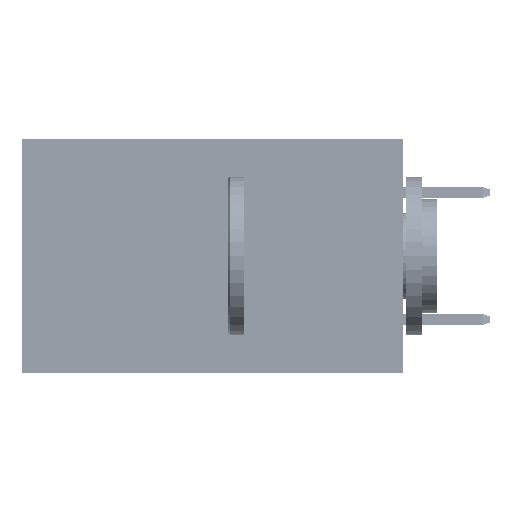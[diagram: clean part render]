
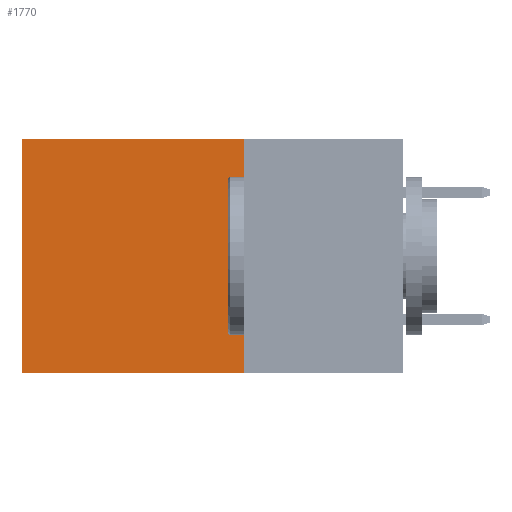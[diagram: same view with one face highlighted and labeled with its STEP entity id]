
A CAD part, left-side view. The second image highlights one B-rep face of the part: STEP entity #1770.
In plain terms, the highlighted planar face has unit normal (-1, 0, 0).
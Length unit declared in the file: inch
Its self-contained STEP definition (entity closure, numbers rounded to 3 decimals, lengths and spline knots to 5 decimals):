
#316 = ORIENTED_EDGE ( 'NONE', *, *, #21267, .F. ) ;
#1166 = CARTESIAN_POINT ( 'NONE',  ( 0.2875, 0.6, -0.37 ) ) ;
#1770 = ADVANCED_FACE ( 'NONE', ( #4336 ), #26639, .F. ) ;
#2137 = CARTESIAN_POINT ( 'NONE',  ( 0.2875, 0.25, -0.37 ) ) ;
#4336 = FACE_OUTER_BOUND ( 'NONE', #8609, .T. ) ;
#5496 = DIRECTION ( 'NONE',  ( 0., 1., 0. ) ) ;
#6066 = VECTOR ( 'NONE', #44348, 39.37008 ) ;
#6526 = AXIS2_PLACEMENT_3D ( 'NONE', #19433, #44395, #40794 ) ;
#7736 = EDGE_CURVE ( 'NONE', #20468, #31080, #27764, .T. ) ;
#8609 = EDGE_LOOP ( 'NONE', ( #12758, #15228, #316, #17844 ) ) ;
#12758 = ORIENTED_EDGE ( 'NONE', *, *, #27454, .T. ) ;
#15228 = ORIENTED_EDGE ( 'NONE', *, *, #7736, .F. ) ;
#17198 = VECTOR ( 'NONE', #45491, 39.37008 ) ;
#17844 = ORIENTED_EDGE ( 'NONE', *, *, #46496, .T. ) ;
#19433 = CARTESIAN_POINT ( 'NONE',  ( 0.2875, 0.25, 0. ) ) ;
#20332 = VECTOR ( 'NONE', #5496, 39.37008 ) ;
#20468 = VERTEX_POINT ( 'NONE', #42370 ) ;
#21267 = EDGE_CURVE ( 'NONE', #22967, #20468, #45347, .T. ) ;
#22967 = VERTEX_POINT ( 'NONE', #47051 ) ;
#22983 = LINE ( 'NONE', #40514, #6066 ) ;
#23268 = CARTESIAN_POINT ( 'NONE',  ( 0.2875, 0.25, 0. ) ) ;
#26639 = PLANE ( 'NONE',  #6526 ) ;
#27454 = EDGE_CURVE ( 'NONE', #29778, #31080, #37834, .T. ) ;
#27764 = LINE ( 'NONE', #2137, #20332 ) ;
#28147 = CARTESIAN_POINT ( 'NONE',  ( 0.2875, 0.6, 0. ) ) ;
#29778 = VERTEX_POINT ( 'NONE', #28147 ) ;
#29816 = DIRECTION ( 'NONE',  ( 0., 0., -1. ) ) ;
#31080 = VERTEX_POINT ( 'NONE', #1166 ) ;
#34460 = CARTESIAN_POINT ( 'NONE',  ( 0.2875, 0.6, 0. ) ) ;
#37834 = LINE ( 'NONE', #34460, #17198 ) ;
#40514 = CARTESIAN_POINT ( 'NONE',  ( 0.2875, 0.25, 0. ) ) ;
#40680 = VECTOR ( 'NONE', #29816, 39.37008 ) ;
#40794 = DIRECTION ( 'NONE',  ( 0., 0., -1. ) ) ;
#42370 = CARTESIAN_POINT ( 'NONE',  ( 0.2875, 0.25, -0.37 ) ) ;
#44348 = DIRECTION ( 'NONE',  ( 0., 1., 0. ) ) ;
#44395 = DIRECTION ( 'NONE',  ( 1., 0., 0. ) ) ;
#45347 = LINE ( 'NONE', #23268, #40680 ) ;
#45491 = DIRECTION ( 'NONE',  ( 0., 0., -1. ) ) ;
#46496 = EDGE_CURVE ( 'NONE', #22967, #29778, #22983, .T. ) ;
#47051 = CARTESIAN_POINT ( 'NONE',  ( 0.2875, 0.25, 0. ) ) ;
